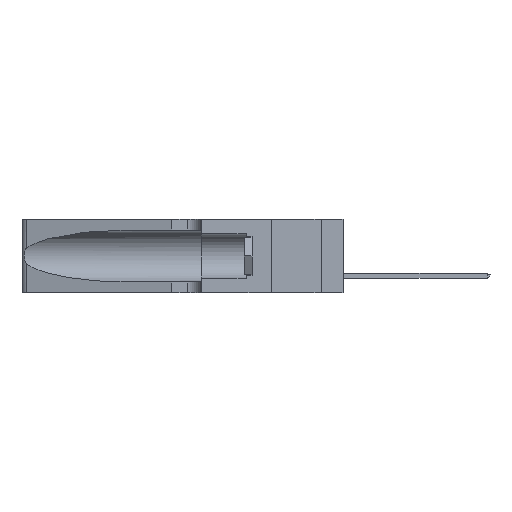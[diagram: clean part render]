
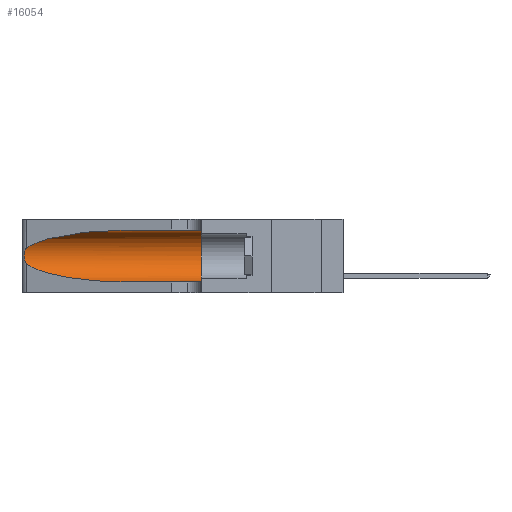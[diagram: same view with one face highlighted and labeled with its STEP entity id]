
A CAD part, left-side view. The second image highlights one B-rep face of the part: STEP entity #16054.
In plain terms, the highlighted cylindrical face has radius 3.308 mm (diameter 6.617 mm), a partial arc.
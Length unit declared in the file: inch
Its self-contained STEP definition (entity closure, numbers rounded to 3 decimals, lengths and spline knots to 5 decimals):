
#3 = VERTEX_POINT ( 'NONE', #27289 ) ;
#262 = CARTESIAN_POINT ( 'NONE',  ( 0.1305, 0.35, 0.31525 ) ) ;
#890 = CARTESIAN_POINT ( 'NONE',  ( 0.25487, 1.22718, 0.14631 ) ) ;
#1426 = CARTESIAN_POINT ( 'NONE',  ( 0.18966, 0.96281, 0.31525 ) ) ;
#1564 = CIRCLE ( 'NONE', #36854, 0.13025 ) ;
#1582 = ORIENTED_EDGE ( 'NONE', *, *, #29282, .T. ) ;
#2212 = CARTESIAN_POINT ( 'NONE',  ( 0.2373, 1.15595, 0.08982 ) ) ;
#2513 = EDGE_LOOP ( 'NONE', ( #1582, #26907, #25031, #35160, #26713, #30120 ) ) ;
#3172 = VERTEX_POINT ( 'NONE', #41209 ) ;
#4147 = CARTESIAN_POINT ( 'NONE',  ( 0.25487, 1.22718, 0.14631 ) ) ;
#4472 = CARTESIAN_POINT ( 'NONE',  ( 0.25639, 1.23184, 0.21858 ) ) ;
#5336 = VERTEX_POINT ( 'NONE', #15831 ) ;
#5819 = FACE_OUTER_BOUND ( 'NONE', #2513, .T. ) ;
#7007 = AXIS2_PLACEMENT_3D ( 'NONE', #22460, #12709, #12109 ) ;
#7559 = CARTESIAN_POINT ( 'NONE',  ( 0.25487, 1.22718, 0.14631 ) ) ;
#7656 = CARTESIAN_POINT ( 'NONE',  ( 0.26018, 1.23835, 0.19895 ) ) ;
#8046 = CARTESIAN_POINT ( 'NONE',  ( 0.2373, 1.15595, 0.28018 ) ) ;
#8359 =( BOUNDED_CURVE ( )  B_SPLINE_CURVE ( 3, ( #4147, #2212, #36082, #42345 ),
 .UNSPECIFIED., .F., .T. ) 
 B_SPLINE_CURVE_WITH_KNOTS ( ( 4, 4 ),
 ( 3.44316, 4.71239 ),
 .UNSPECIFIED. ) 
 CURVE ( )  GEOMETRIC_REPRESENTATION_ITEM ( )  RATIONAL_B_SPLINE_CURVE ( ( 1., 0.87, 0.87, 1. ) ) 
 REPRESENTATION_ITEM ( '' )  );
#11088 = CARTESIAN_POINT ( 'NONE',  ( 0.25856, 1.23593, 0.16098 ) ) ;
#11183 = CARTESIAN_POINT ( 'NONE',  ( 0.25487, 1.22718, 0.22369 ) ) ;
#11519 = CARTESIAN_POINT ( 'NONE',  ( 0.1305, 1.61858, 0.05475 ) ) ;
#11667 = B_SPLINE_CURVE_WITH_KNOTS ( 'NONE', 3,
 ( #24746, #38718, #4472, #41961, #28170, #7656, #38578, #31621, #28496, #11088, #35085, #18023, #21451, #890 ),
 .UNSPECIFIED., .F., .F.,
 ( 4, 2, 2, 2, 2, 2, 4 ),
 ( 0., 0.00027, 0.00053, 0.00107, 0.0016, 0.00187, 0.00214 ),
 .UNSPECIFIED. ) ;
#12109 = DIRECTION ( 'NONE',  ( 0., 0., -1. ) ) ;
#12709 = DIRECTION ( 'NONE',  ( 0., -1., 0. ) ) ;
#13574 = DIRECTION ( 'NONE',  ( 0., 1., 0. ) ) ;
#14420 =( BOUNDED_CURVE ( )  B_SPLINE_CURVE ( 3, ( #39257, #1426, #8046, #11183 ),
 .UNSPECIFIED., .F., .F. ) 
 B_SPLINE_CURVE_WITH_KNOTS ( ( 4, 4 ),
 ( 1.5708, 2.84003 ),
 .UNSPECIFIED. ) 
 CURVE ( )  GEOMETRIC_REPRESENTATION_ITEM ( )  RATIONAL_B_SPLINE_CURVE ( ( 1., 0.87, 0.87, 1. ) ) 
 REPRESENTATION_ITEM ( '' )  );
#14998 = EDGE_CURVE ( 'NONE', #16307, #29458, #8359, .T. ) ;
#15831 = CARTESIAN_POINT ( 'NONE',  ( 0.25487, 1.22718, 0.22369 ) ) ;
#16054 = ADVANCED_FACE ( 'NONE', ( #5819 ), #33708, .F. ) ;
#16307 = VERTEX_POINT ( 'NONE', #7559 ) ;
#17258 = CARTESIAN_POINT ( 'NONE',  ( 0.1305, 0.72297, 0.05475 ) ) ;
#18023 = CARTESIAN_POINT ( 'NONE',  ( 0.25639, 1.23186, 0.15144 ) ) ;
#18584 = DIRECTION ( 'NONE',  ( 0., -1., 0. ) ) ;
#19308 = VECTOR ( 'NONE', #37359, 39.37008 ) ;
#20539 = VERTEX_POINT ( 'NONE', #262 ) ;
#21451 = CARTESIAN_POINT ( 'NONE',  ( 0.25555, 1.22993, 0.14849 ) ) ;
#22460 = CARTESIAN_POINT ( 'NONE',  ( 0.1305, 1.61858, 0.185 ) ) ;
#24746 = CARTESIAN_POINT ( 'NONE',  ( 0.25487, 1.22718, 0.22369 ) ) ;
#25031 = ORIENTED_EDGE ( 'NONE', *, *, #14998, .T. ) ;
#25268 = VECTOR ( 'NONE', #18584, 39.37008 ) ;
#26713 = ORIENTED_EDGE ( 'NONE', *, *, #42656, .F. ) ;
#26907 = ORIENTED_EDGE ( 'NONE', *, *, #32807, .T. ) ;
#27289 = CARTESIAN_POINT ( 'NONE',  ( 0.1305, 0.72297, 0.31525 ) ) ;
#28170 = CARTESIAN_POINT ( 'NONE',  ( 0.25854, 1.2359, 0.20912 ) ) ;
#28496 = CARTESIAN_POINT ( 'NONE',  ( 0.26017, 1.23833, 0.17102 ) ) ;
#29282 = EDGE_CURVE ( 'NONE', #3, #5336, #14420, .T. ) ;
#29458 = VERTEX_POINT ( 'NONE', #17258 ) ;
#30120 = ORIENTED_EDGE ( 'NONE', *, *, #42210, .F. ) ;
#31621 = CARTESIAN_POINT ( 'NONE',  ( 0.26075, 1.23896, 0.178 ) ) ;
#32807 = EDGE_CURVE ( 'NONE', #5336, #16307, #11667, .T. ) ;
#33708 = CYLINDRICAL_SURFACE ( 'NONE', #7007, 0.13025 ) ;
#35085 = CARTESIAN_POINT ( 'NONE',  ( 0.25789, 1.23486, 0.15765 ) ) ;
#35160 = ORIENTED_EDGE ( 'NONE', *, *, #40726, .T. ) ;
#36082 = CARTESIAN_POINT ( 'NONE',  ( 0.18966, 0.96281, 0.05475 ) ) ;
#36854 = AXIS2_PLACEMENT_3D ( 'NONE', #44401, #13574, #37697 ) ;
#37359 = DIRECTION ( 'NONE',  ( 0., -1., 0. ) ) ;
#37697 = DIRECTION ( 'NONE',  ( 0., 0., 1. ) ) ;
#38578 = CARTESIAN_POINT ( 'NONE',  ( 0.26075, 1.23896, 0.19203 ) ) ;
#38718 = CARTESIAN_POINT ( 'NONE',  ( 0.25555, 1.22994, 0.2215 ) ) ;
#39257 = CARTESIAN_POINT ( 'NONE',  ( 0.1305, 0.72297, 0.31525 ) ) ;
#40726 = EDGE_CURVE ( 'NONE', #29458, #3172, #43494, .T. ) ;
#41073 = CARTESIAN_POINT ( 'NONE',  ( 0.1305, 1.61858, 0.31525 ) ) ;
#41209 = CARTESIAN_POINT ( 'NONE',  ( 0.1305, 0.35, 0.05475 ) ) ;
#41961 = CARTESIAN_POINT ( 'NONE',  ( 0.25787, 1.23484, 0.2124 ) ) ;
#42210 = EDGE_CURVE ( 'NONE', #3, #20539, #43939, .T. ) ;
#42345 = CARTESIAN_POINT ( 'NONE',  ( 0.1305, 0.72297, 0.05475 ) ) ;
#42656 = EDGE_CURVE ( 'NONE', #20539, #3172, #1564, .T. ) ;
#43494 = LINE ( 'NONE', #11519, #25268 ) ;
#43939 = LINE ( 'NONE', #41073, #19308 ) ;
#44401 = CARTESIAN_POINT ( 'NONE',  ( 0.1305, 0.35, 0.185 ) ) ;
